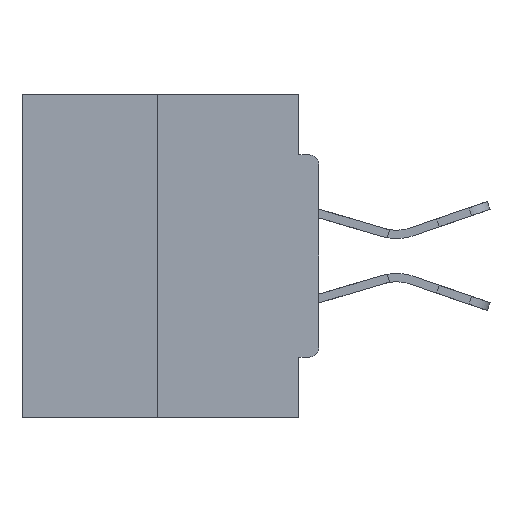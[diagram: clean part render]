
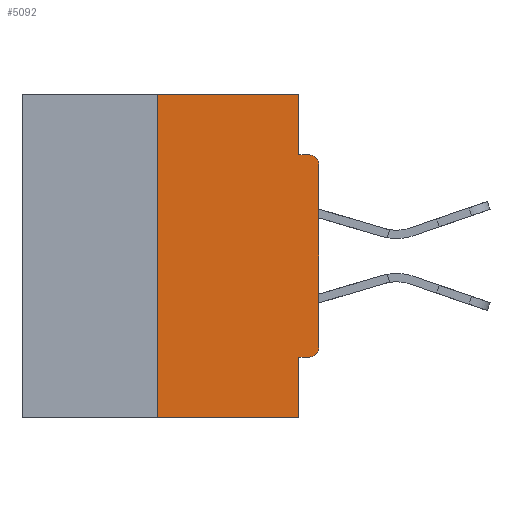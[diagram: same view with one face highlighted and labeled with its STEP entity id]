
A CAD part, left-side view. The second image highlights one B-rep face of the part: STEP entity #5092.
In plain terms, the highlighted planar face has unit normal (-1, 0, 0).
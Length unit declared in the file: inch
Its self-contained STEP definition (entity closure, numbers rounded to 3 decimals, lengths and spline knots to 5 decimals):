
#2279 = ORIENTED_EDGE ( 'NONE', *, *, #36434, .T. ) ;
#2809 = CARTESIAN_POINT ( 'NONE',  ( 0., 0., 0. ) ) ;
#3046 = CARTESIAN_POINT ( 'NONE',  ( 0., 0.25, -0.5 ) ) ;
#3533 = LINE ( 'NONE', #18656, #12197 ) ;
#3626 = DIRECTION ( 'NONE',  ( 0., -1., 0. ) ) ;
#3634 = EDGE_CURVE ( 'NONE', #22701, #22697, #11146, .T. ) ;
#3844 = VERTEX_POINT ( 'NONE', #31763 ) ;
#4017 = VECTOR ( 'NONE', #9989, 39.37008 ) ;
#4156 = VERTEX_POINT ( 'NONE', #34495 ) ;
#4418 = CARTESIAN_POINT ( 'NONE',  ( 0., 0.015, -0.1085 ) ) ;
#5092 = ADVANCED_FACE ( 'NONE', ( #10463 ), #30386, .F. ) ;
#5807 = VERTEX_POINT ( 'NONE', #17512 ) ;
#6434 = CARTESIAN_POINT ( 'NONE',  ( 0., 0.46, 0. ) ) ;
#8682 = VERTEX_POINT ( 'NONE', #38090 ) ;
#9989 = DIRECTION ( 'NONE',  ( 0., 0., -1. ) ) ;
#10463 = FACE_OUTER_BOUND ( 'NONE', #41483, .T. ) ;
#10601 = ORIENTED_EDGE ( 'NONE', *, *, #31949, .F. ) ;
#10767 = VERTEX_POINT ( 'NONE', #22493 ) ;
#10966 = EDGE_CURVE ( 'NONE', #4156, #10767, #37977, .T. ) ;
#11146 = LINE ( 'NONE', #26442, #12810 ) ;
#12109 = EDGE_CURVE ( 'NONE', #5807, #10767, #26024, .T. ) ;
#12197 = VECTOR ( 'NONE', #18204, 39.37008 ) ;
#12799 = CARTESIAN_POINT ( 'NONE',  ( 0., 0.031, -0.5 ) ) ;
#12810 = VECTOR ( 'NONE', #19387, 39.37008 ) ;
#13417 = DIRECTION ( 'NONE',  ( 0., 0., -1. ) ) ;
#14034 = CARTESIAN_POINT ( 'NONE',  ( 0., 0.015, -0.3915 ) ) ;
#15676 = LINE ( 'NONE', #19310, #37166 ) ;
#16065 = DIRECTION ( 'NONE',  ( 0., 0., 1. ) ) ;
#16234 = VECTOR ( 'NONE', #16065, 39.37008 ) ;
#17286 = ORIENTED_EDGE ( 'NONE', *, *, #37429, .F. ) ;
#17341 = ORIENTED_EDGE ( 'NONE', *, *, #10966, .F. ) ;
#17512 = CARTESIAN_POINT ( 'NONE',  ( 0., 0., -0.1085 ) ) ;
#18077 = EDGE_CURVE ( 'NONE', #8682, #33917, #37079, .T. ) ;
#18204 = DIRECTION ( 'NONE',  ( 0., -1., 0. ) ) ;
#18555 = ORIENTED_EDGE ( 'NONE', *, *, #3634, .F. ) ;
#18656 = CARTESIAN_POINT ( 'NONE',  ( 0., 0.46, -0.5 ) ) ;
#18762 = DIRECTION ( 'NONE',  ( 0., 1., 0. ) ) ;
#19310 = CARTESIAN_POINT ( 'NONE',  ( 0., 0.031, -0.5 ) ) ;
#19387 = DIRECTION ( 'NONE',  ( 0., 0., 1. ) ) ;
#19715 = VECTOR ( 'NONE', #32517, 39.37008 ) ;
#19807 = EDGE_CURVE ( 'NONE', #22701, #35262, #3533, .T. ) ;
#20043 = DIRECTION ( 'NONE',  ( 1., 0., 0. ) ) ;
#20273 = EDGE_CURVE ( 'NONE', #38396, #4156, #43348, .T. ) ;
#21751 = DIRECTION ( 'NONE',  ( -1., 0., 0. ) ) ;
#22493 = CARTESIAN_POINT ( 'NONE',  ( 0., 0.015, -0.0935 ) ) ;
#22697 = VERTEX_POINT ( 'NONE', #27264 ) ;
#22701 = VERTEX_POINT ( 'NONE', #3046 ) ;
#22905 = LINE ( 'NONE', #29081, #19715 ) ;
#23168 = LINE ( 'NONE', #2809, #16234 ) ;
#23520 = CARTESIAN_POINT ( 'NONE',  ( 0., 0.031, 0. ) ) ;
#24413 = ORIENTED_EDGE ( 'NONE', *, *, #20273, .F. ) ;
#25482 = CARTESIAN_POINT ( 'NONE',  ( 0., 0.031, -0.4065 ) ) ;
#26024 = CIRCLE ( 'NONE', #43538, 0.015 ) ;
#26442 = CARTESIAN_POINT ( 'NONE',  ( 0., 0.25, 0. ) ) ;
#27264 = CARTESIAN_POINT ( 'NONE',  ( 0., 0.25, 0. ) ) ;
#28694 = CARTESIAN_POINT ( 'NONE',  ( 0., 0., -0.4065 ) ) ;
#29081 = CARTESIAN_POINT ( 'NONE',  ( 0., 0.46, 0. ) ) ;
#30386 = PLANE ( 'NONE',  #36968 ) ;
#30674 = ORIENTED_EDGE ( 'NONE', *, *, #30864, .T. ) ;
#30864 = EDGE_CURVE ( 'NONE', #3844, #5807, #23168, .T. ) ;
#30885 = CARTESIAN_POINT ( 'NONE',  ( 0., 0., -0.0935 ) ) ;
#31139 = DIRECTION ( 'NONE',  ( -1., 0., 0. ) ) ;
#31763 = CARTESIAN_POINT ( 'NONE',  ( 0., 0., -0.3915 ) ) ;
#31949 = EDGE_CURVE ( 'NONE', #33917, #35262, #15676, .T. ) ;
#31957 = DIRECTION ( 'NONE',  ( 0., 0., -1. ) ) ;
#32517 = DIRECTION ( 'NONE',  ( 0., -1., 0. ) ) ;
#33917 = VERTEX_POINT ( 'NONE', #25482 ) ;
#34131 = ORIENTED_EDGE ( 'NONE', *, *, #12109, .T. ) ;
#34394 = ORIENTED_EDGE ( 'NONE', *, *, #18077, .F. ) ;
#34495 = CARTESIAN_POINT ( 'NONE',  ( 0., 0.031, -0.0935 ) ) ;
#35262 = VERTEX_POINT ( 'NONE', #12799 ) ;
#35802 = VECTOR ( 'NONE', #3626, 39.37008 ) ;
#36434 = EDGE_CURVE ( 'NONE', #8682, #3844, #39441, .T. ) ;
#36968 = AXIS2_PLACEMENT_3D ( 'NONE', #6434, #20043, #13417 ) ;
#37079 = LINE ( 'NONE', #28694, #39788 ) ;
#37166 = VECTOR ( 'NONE', #43987, 39.37008 ) ;
#37429 = EDGE_CURVE ( 'NONE', #22697, #38396, #22905, .T. ) ;
#37977 = LINE ( 'NONE', #30885, #35802 ) ;
#38090 = CARTESIAN_POINT ( 'NONE',  ( 0., 0.015, -0.4065 ) ) ;
#38396 = VERTEX_POINT ( 'NONE', #39660 ) ;
#39441 = CIRCLE ( 'NONE', #40562, 0.015 ) ;
#39660 = CARTESIAN_POINT ( 'NONE',  ( 0., 0.031, 0. ) ) ;
#39788 = VECTOR ( 'NONE', #18762, 39.37008 ) ;
#40562 = AXIS2_PLACEMENT_3D ( 'NONE', #14034, #31139, #41536 ) ;
#41483 = EDGE_LOOP ( 'NONE', ( #17286, #18555, #42301, #10601, #34394, #2279, #30674, #34131, #17341, #24413 ) ) ;
#41536 = DIRECTION ( 'NONE',  ( 0., 0., -1. ) ) ;
#42301 = ORIENTED_EDGE ( 'NONE', *, *, #19807, .T. ) ;
#43348 = LINE ( 'NONE', #23520, #4017 ) ;
#43538 = AXIS2_PLACEMENT_3D ( 'NONE', #4418, #21751, #31957 ) ;
#43987 = DIRECTION ( 'NONE',  ( 0., 0., -1. ) ) ;
